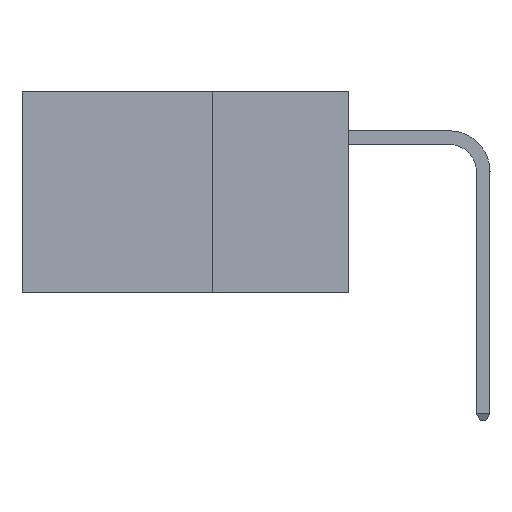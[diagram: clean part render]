
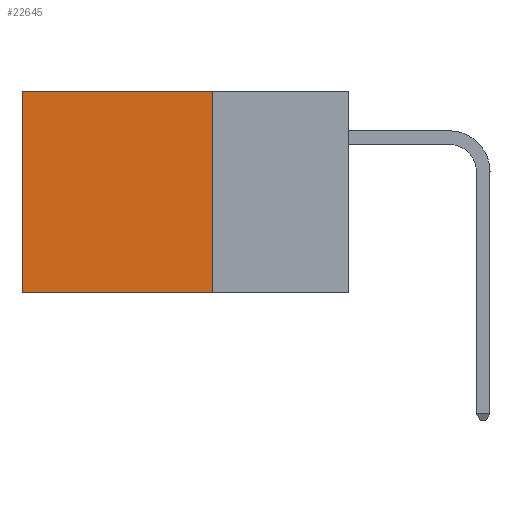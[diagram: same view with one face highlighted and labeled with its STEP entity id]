
A CAD part, left-side view. The second image highlights one B-rep face of the part: STEP entity #22645.
In plain terms, the highlighted planar face has unit normal (-1, 0, 0).
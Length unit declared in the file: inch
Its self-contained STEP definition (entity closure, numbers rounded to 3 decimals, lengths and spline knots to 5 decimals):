
#3100 = EDGE_CURVE ( 'NONE', #38316, #9717, #25602, .T. ) ;
#6077 = VERTEX_POINT ( 'NONE', #37075 ) ;
#9717 = VERTEX_POINT ( 'NONE', #21423 ) ;
#10088 = VECTOR ( 'NONE', #38426, 39.37008 ) ;
#10503 = CARTESIAN_POINT ( 'NONE',  ( 0.2875, 0.6, 0. ) ) ;
#12042 = LINE ( 'NONE', #19157, #27479 ) ;
#13566 = ORIENTED_EDGE ( 'NONE', *, *, #32189, .T. ) ;
#14525 = DIRECTION ( 'NONE',  ( 1., 0., 0. ) ) ;
#15231 = EDGE_CURVE ( 'NONE', #6077, #15400, #12042, .T. ) ;
#15400 = VERTEX_POINT ( 'NONE', #10503 ) ;
#15608 = ORIENTED_EDGE ( 'NONE', *, *, #3100, .F. ) ;
#16457 = VECTOR ( 'NONE', #23371, 39.37008 ) ;
#17358 = CARTESIAN_POINT ( 'NONE',  ( 0.2875, 0.25, 0. ) ) ;
#19157 = CARTESIAN_POINT ( 'NONE',  ( 0.2875, 0.25, 0. ) ) ;
#21423 = CARTESIAN_POINT ( 'NONE',  ( 0.2875, 0.6, -0.37 ) ) ;
#21480 = AXIS2_PLACEMENT_3D ( 'NONE', #32806, #14525, #35825 ) ;
#22203 = DIRECTION ( 'NONE',  ( 0., 1., 0. ) ) ;
#22267 = LINE ( 'NONE', #24377, #37350 ) ;
#22645 = ADVANCED_FACE ( 'NONE', ( #26421 ), #29789, .F. ) ;
#23371 = DIRECTION ( 'NONE',  ( 0., 0., -1. ) ) ;
#24377 = CARTESIAN_POINT ( 'NONE',  ( 0.2875, 0.6, 0. ) ) ;
#25602 = LINE ( 'NONE', #38452, #10088 ) ;
#26421 = FACE_OUTER_BOUND ( 'NONE', #39563, .T. ) ;
#26910 = ORIENTED_EDGE ( 'NONE', *, *, #36358, .F. ) ;
#27419 = DIRECTION ( 'NONE',  ( 0., 0., -1. ) ) ;
#27479 = VECTOR ( 'NONE', #22203, 39.37008 ) ;
#29789 = PLANE ( 'NONE',  #21480 ) ;
#32189 = EDGE_CURVE ( 'NONE', #15400, #9717, #22267, .T. ) ;
#32806 = CARTESIAN_POINT ( 'NONE',  ( 0.2875, 0.25, 0. ) ) ;
#33654 = CARTESIAN_POINT ( 'NONE',  ( 0.2875, 0.25, -0.37 ) ) ;
#35825 = DIRECTION ( 'NONE',  ( 0., 0., -1. ) ) ;
#36358 = EDGE_CURVE ( 'NONE', #6077, #38316, #39633, .T. ) ;
#37075 = CARTESIAN_POINT ( 'NONE',  ( 0.2875, 0.25, 0. ) ) ;
#37277 = ORIENTED_EDGE ( 'NONE', *, *, #15231, .T. ) ;
#37350 = VECTOR ( 'NONE', #27419, 39.37008 ) ;
#38316 = VERTEX_POINT ( 'NONE', #33654 ) ;
#38426 = DIRECTION ( 'NONE',  ( 0., 1., 0. ) ) ;
#38452 = CARTESIAN_POINT ( 'NONE',  ( 0.2875, 0.25, -0.37 ) ) ;
#39563 = EDGE_LOOP ( 'NONE', ( #13566, #15608, #26910, #37277 ) ) ;
#39633 = LINE ( 'NONE', #17358, #16457 ) ;
